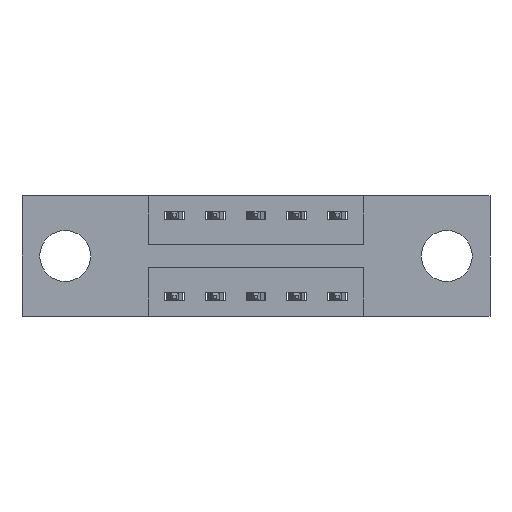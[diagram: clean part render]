
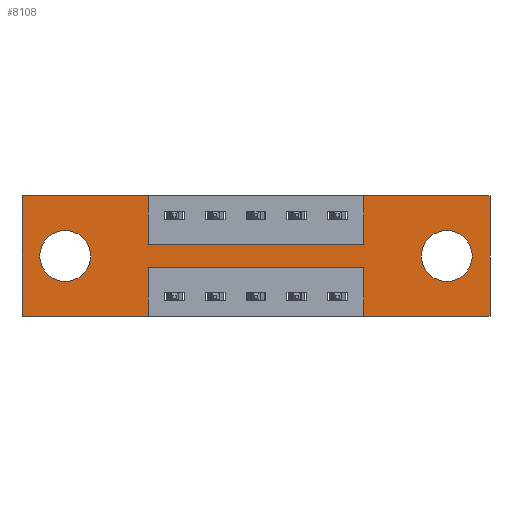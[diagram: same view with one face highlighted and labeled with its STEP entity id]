
A CAD part, front view. The second image highlights one B-rep face of the part: STEP entity #8108.
In plain terms, the highlighted planar face has unit normal (0, -1, 0).
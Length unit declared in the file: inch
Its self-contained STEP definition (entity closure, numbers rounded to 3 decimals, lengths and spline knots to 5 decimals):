
#28 = EDGE_CURVE ( 'NONE', #3569, #5031, #6473, .T. ) ;
#35 = VECTOR ( 'NONE', #1855, 39.37008 ) ;
#246 = CARTESIAN_POINT ( 'NONE',  ( 0., 0., -0.37 ) ) ;
#256 = CARTESIAN_POINT ( 'NONE',  ( 0.1325, 0., -0.263 ) ) ;
#265 = ORIENTED_EDGE ( 'NONE', *, *, #3520, .F. ) ;
#266 = CARTESIAN_POINT ( 'NONE',  ( 1.3025, 0., -0.263 ) ) ;
#313 = LINE ( 'NONE', #6695, #2711 ) ;
#383 = EDGE_LOOP ( 'NONE', ( #2776, #4436 ) ) ;
#466 = VECTOR ( 'NONE', #6137, 39.37008 ) ;
#482 = ORIENTED_EDGE ( 'NONE', *, *, #600, .F. ) ;
#537 = AXIS2_PLACEMENT_3D ( 'NONE', #881, #6633, #968 ) ;
#591 = VERTEX_POINT ( 'NONE', #7326 ) ;
#600 = EDGE_CURVE ( 'NONE', #5031, #7841, #6174, .T. ) ;
#649 = ORIENTED_EDGE ( 'NONE', *, *, #940, .F. ) ;
#714 = LINE ( 'NONE', #6517, #2923 ) ;
#768 = LINE ( 'NONE', #3491, #2277 ) ;
#844 = EDGE_LOOP ( 'NONE', ( #8259, #4488 ) ) ;
#849 = DIRECTION ( 'NONE',  ( 0., 0., -1. ) ) ;
#881 = CARTESIAN_POINT ( 'NONE',  ( 0.1325, 0., -0.185 ) ) ;
#896 = CARTESIAN_POINT ( 'NONE',  ( 1.3025, 0., -0.185 ) ) ;
#940 = EDGE_CURVE ( 'NONE', #5848, #1939, #2275, .T. ) ;
#957 = ORIENTED_EDGE ( 'NONE', *, *, #7093, .F. ) ;
#968 = DIRECTION ( 'NONE',  ( 0., 0., 1. ) ) ;
#970 = DIRECTION ( 'NONE',  ( -1., 0., 0. ) ) ;
#996 = CARTESIAN_POINT ( 'NONE',  ( 1.0475, 0., -0.22 ) ) ;
#1031 = CARTESIAN_POINT ( 'NONE',  ( 0., 0., 0. ) ) ;
#1059 = LINE ( 'NONE', #2080, #6040 ) ;
#1133 = AXIS2_PLACEMENT_3D ( 'NONE', #3239, #6468, #7746 ) ;
#1175 = CARTESIAN_POINT ( 'NONE',  ( 0.3875, 0., -0.22 ) ) ;
#1384 = AXIS2_PLACEMENT_3D ( 'NONE', #896, #1562, #6647 ) ;
#1480 = CARTESIAN_POINT ( 'NONE',  ( 0., 0., 0. ) ) ;
#1496 = VERTEX_POINT ( 'NONE', #5367 ) ;
#1562 = DIRECTION ( 'NONE',  ( 0., 1., 0. ) ) ;
#1598 = CARTESIAN_POINT ( 'NONE',  ( 0.3875, 0., -0.15 ) ) ;
#1617 = CARTESIAN_POINT ( 'NONE',  ( 0.3875, 0., -0.37 ) ) ;
#1855 = DIRECTION ( 'NONE',  ( 1., 0., 0. ) ) ;
#1939 = VERTEX_POINT ( 'NONE', #1480 ) ;
#2080 = CARTESIAN_POINT ( 'NONE',  ( 1.435, 0., 0. ) ) ;
#2239 = ORIENTED_EDGE ( 'NONE', *, *, #6669, .F. ) ;
#2275 = LINE ( 'NONE', #1031, #466 ) ;
#2276 = AXIS2_PLACEMENT_3D ( 'NONE', #246, #6029, #3364 ) ;
#2277 = VECTOR ( 'NONE', #8250, 39.37008 ) ;
#2315 = DIRECTION ( 'NONE',  ( 0., 0., 1. ) ) ;
#2572 = VERTEX_POINT ( 'NONE', #256 ) ;
#2706 = ORIENTED_EDGE ( 'NONE', *, *, #7162, .F. ) ;
#2711 = VECTOR ( 'NONE', #849, 39.37008 ) ;
#2744 = CARTESIAN_POINT ( 'NONE',  ( 0.3875, 0., 0. ) ) ;
#2765 = VECTOR ( 'NONE', #4484, 39.37008 ) ;
#2776 = ORIENTED_EDGE ( 'NONE', *, *, #5053, .T. ) ;
#2780 = FACE_OUTER_BOUND ( 'NONE', #7977, .T. ) ;
#2792 = DIRECTION ( 'NONE',  ( -1., 0., 0. ) ) ;
#2797 = VERTEX_POINT ( 'NONE', #6308 ) ;
#2883 = CARTESIAN_POINT ( 'NONE',  ( 1.0475, 0., -0.37 ) ) ;
#2923 = VECTOR ( 'NONE', #3376, 39.37008 ) ;
#3072 = CIRCLE ( 'NONE', #537, 0.078 ) ;
#3102 = VECTOR ( 'NONE', #3132, 39.37008 ) ;
#3132 = DIRECTION ( 'NONE',  ( 0., 0., -1. ) ) ;
#3138 = ORIENTED_EDGE ( 'NONE', *, *, #3473, .F. ) ;
#3188 = CARTESIAN_POINT ( 'NONE',  ( 0., 0., 0. ) ) ;
#3204 = EDGE_CURVE ( 'NONE', #591, #7260, #6775, .T. ) ;
#3239 = CARTESIAN_POINT ( 'NONE',  ( 0.1325, 0., -0.185 ) ) ;
#3302 = CARTESIAN_POINT ( 'NONE',  ( 0.3875, 0., -0.15 ) ) ;
#3316 = EDGE_CURVE ( 'NONE', #1939, #3878, #768, .T. ) ;
#3342 = AXIS2_PLACEMENT_3D ( 'NONE', #5516, #5482, #5690 ) ;
#3364 = DIRECTION ( 'NONE',  ( 0., 0., -1. ) ) ;
#3376 = DIRECTION ( 'NONE',  ( -1., 0., 0. ) ) ;
#3439 = CARTESIAN_POINT ( 'NONE',  ( 1.0475, 0., 0. ) ) ;
#3473 = EDGE_CURVE ( 'NONE', #3624, #7096, #1059, .T. ) ;
#3489 = CARTESIAN_POINT ( 'NONE',  ( 0., 0., -0.37 ) ) ;
#3491 = CARTESIAN_POINT ( 'NONE',  ( 0., 0., 0. ) ) ;
#3520 = EDGE_CURVE ( 'NONE', #7096, #3569, #4065, .T. ) ;
#3569 = VERTEX_POINT ( 'NONE', #2883 ) ;
#3624 = VERTEX_POINT ( 'NONE', #4017 ) ;
#3878 = VERTEX_POINT ( 'NONE', #2744 ) ;
#4017 = CARTESIAN_POINT ( 'NONE',  ( 1.435, 0., 0. ) ) ;
#4044 = CARTESIAN_POINT ( 'NONE',  ( 1.0475, 0., -0.37 ) ) ;
#4065 = LINE ( 'NONE', #3489, #4178 ) ;
#4086 = VECTOR ( 'NONE', #2792, 39.37008 ) ;
#4178 = VECTOR ( 'NONE', #970, 39.37008 ) ;
#4305 = VERTEX_POINT ( 'NONE', #3439 ) ;
#4326 = EDGE_CURVE ( 'NONE', #7260, #591, #4962, .T. ) ;
#4398 = VERTEX_POINT ( 'NONE', #1598 ) ;
#4436 = ORIENTED_EDGE ( 'NONE', *, *, #6462, .T. ) ;
#4484 = DIRECTION ( 'NONE',  ( 0., 0., 1. ) ) ;
#4488 = ORIENTED_EDGE ( 'NONE', *, *, #4326, .T. ) ;
#4597 = ORIENTED_EDGE ( 'NONE', *, *, #28, .F. ) ;
#4657 = EDGE_CURVE ( 'NONE', #7841, #4921, #4790, .T. ) ;
#4790 = LINE ( 'NONE', #8049, #3102 ) ;
#4806 = CARTESIAN_POINT ( 'NONE',  ( 0.3875, 0., -0.22 ) ) ;
#4897 = ORIENTED_EDGE ( 'NONE', *, *, #7615, .F. ) ;
#4921 = VERTEX_POINT ( 'NONE', #1617 ) ;
#4962 = CIRCLE ( 'NONE', #1384, 0.078 ) ;
#5031 = VERTEX_POINT ( 'NONE', #996 ) ;
#5053 = EDGE_CURVE ( 'NONE', #2797, #2572, #3072, .T. ) ;
#5367 = CARTESIAN_POINT ( 'NONE',  ( 1.0475, 0., -0.15 ) ) ;
#5482 = DIRECTION ( 'NONE',  ( 0., 1., 0. ) ) ;
#5516 = CARTESIAN_POINT ( 'NONE',  ( 1.3025, 0., -0.185 ) ) ;
#5576 = FACE_BOUND ( 'NONE', #383, .T. ) ;
#5634 = CIRCLE ( 'NONE', #1133, 0.078 ) ;
#5690 = DIRECTION ( 'NONE',  ( 0., 0., -1. ) ) ;
#5848 = VERTEX_POINT ( 'NONE', #7909 ) ;
#5889 = PLANE ( 'NONE',  #2276 ) ;
#5944 = ORIENTED_EDGE ( 'NONE', *, *, #6310, .F. ) ;
#6029 = DIRECTION ( 'NONE',  ( 0., -1., 0. ) ) ;
#6040 = VECTOR ( 'NONE', #8042, 39.37008 ) ;
#6137 = DIRECTION ( 'NONE',  ( 0., 0., 1. ) ) ;
#6174 = LINE ( 'NONE', #4806, #4086 ) ;
#6278 = LINE ( 'NONE', #8275, #2765 ) ;
#6285 = VECTOR ( 'NONE', #2315, 39.37008 ) ;
#6308 = CARTESIAN_POINT ( 'NONE',  ( 0.1325, 0., -0.107 ) ) ;
#6310 = EDGE_CURVE ( 'NONE', #4305, #3624, #6446, .T. ) ;
#6325 = ORIENTED_EDGE ( 'NONE', *, *, #4657, .F. ) ;
#6351 = VECTOR ( 'NONE', #7768, 39.37008 ) ;
#6446 = LINE ( 'NONE', #3188, #35 ) ;
#6462 = EDGE_CURVE ( 'NONE', #2572, #2797, #5634, .T. ) ;
#6468 = DIRECTION ( 'NONE',  ( 0., 1., 0. ) ) ;
#6473 = LINE ( 'NONE', #4044, #6285 ) ;
#6517 = CARTESIAN_POINT ( 'NONE',  ( 0., 0., -0.37 ) ) ;
#6633 = DIRECTION ( 'NONE',  ( 0., 1., 0. ) ) ;
#6647 = DIRECTION ( 'NONE',  ( 0., 0., -1. ) ) ;
#6669 = EDGE_CURVE ( 'NONE', #3878, #4398, #313, .T. ) ;
#6695 = CARTESIAN_POINT ( 'NONE',  ( 0.3875, 0., 0. ) ) ;
#6775 = CIRCLE ( 'NONE', #3342, 0.078 ) ;
#7093 = EDGE_CURVE ( 'NONE', #1496, #4305, #6278, .T. ) ;
#7096 = VERTEX_POINT ( 'NONE', #7102 ) ;
#7102 = CARTESIAN_POINT ( 'NONE',  ( 1.435, 0., -0.37 ) ) ;
#7162 = EDGE_CURVE ( 'NONE', #4398, #1496, #8032, .T. ) ;
#7260 = VERTEX_POINT ( 'NONE', #266 ) ;
#7326 = CARTESIAN_POINT ( 'NONE',  ( 1.3025, 0., -0.107 ) ) ;
#7392 = FACE_BOUND ( 'NONE', #844, .T. ) ;
#7615 = EDGE_CURVE ( 'NONE', #4921, #5848, #714, .T. ) ;
#7746 = DIRECTION ( 'NONE',  ( 0., 0., 1. ) ) ;
#7768 = DIRECTION ( 'NONE',  ( 1., 0., 0. ) ) ;
#7841 = VERTEX_POINT ( 'NONE', #1175 ) ;
#7903 = ORIENTED_EDGE ( 'NONE', *, *, #3316, .F. ) ;
#7909 = CARTESIAN_POINT ( 'NONE',  ( 0., 0., -0.37 ) ) ;
#7977 = EDGE_LOOP ( 'NONE', ( #6325, #482, #4597, #265, #3138, #5944, #957, #2706, #2239, #7903, #649, #4897 ) ) ;
#8032 = LINE ( 'NONE', #3302, #6351 ) ;
#8042 = DIRECTION ( 'NONE',  ( 0., 0., -1. ) ) ;
#8049 = CARTESIAN_POINT ( 'NONE',  ( 0.3875, 0., -0.37 ) ) ;
#8108 = ADVANCED_FACE ( 'NONE', ( #7392, #5576, #2780 ), #5889, .T. ) ;
#8250 = DIRECTION ( 'NONE',  ( 1., 0., 0. ) ) ;
#8259 = ORIENTED_EDGE ( 'NONE', *, *, #3204, .T. ) ;
#8275 = CARTESIAN_POINT ( 'NONE',  ( 1.0475, 0., 0. ) ) ;
